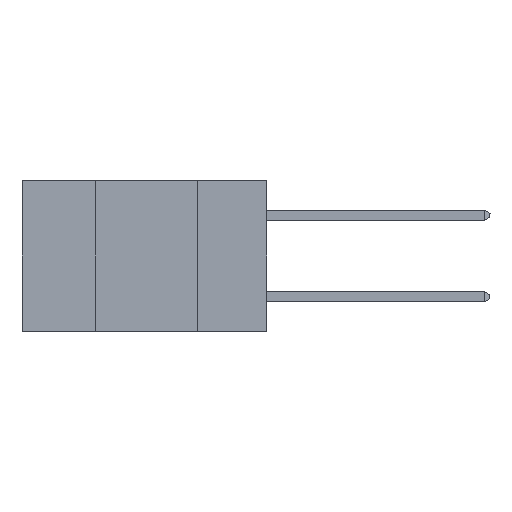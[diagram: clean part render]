
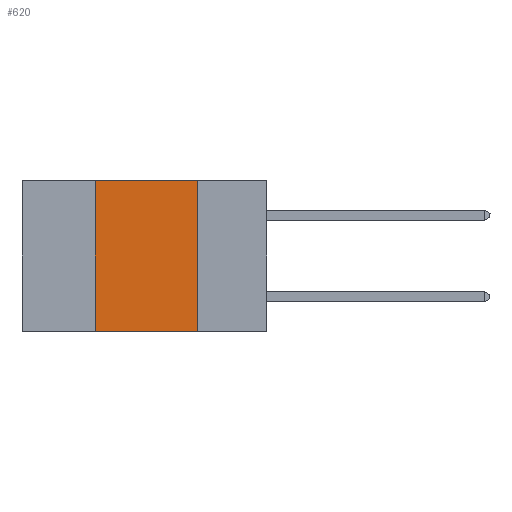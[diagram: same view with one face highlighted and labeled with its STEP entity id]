
A CAD part, left-side view. The second image highlights one B-rep face of the part: STEP entity #620.
In plain terms, the highlighted planar face has unit normal (-1, 0, 0).
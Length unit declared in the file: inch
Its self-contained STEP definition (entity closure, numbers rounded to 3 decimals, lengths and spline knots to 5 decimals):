
#140 = EDGE_CURVE ( 'NONE', #12637, #9687, #12186, .T. ) ;
#423 = EDGE_LOOP ( 'NONE', ( #9757, #9960, #8220, #6773 ) ) ;
#484 = CARTESIAN_POINT ( 'NONE',  ( 0., 0.42, -0.37 ) ) ;
#620 = ADVANCED_FACE ( 'NONE', ( #1312 ), #9565, .F. ) ;
#869 = EDGE_CURVE ( 'NONE', #1487, #12637, #4148, .T. ) ;
#1088 = CARTESIAN_POINT ( 'NONE',  ( 0., 0.17, 0. ) ) ;
#1160 = CARTESIAN_POINT ( 'NONE',  ( 0., 0.17, -0.37 ) ) ;
#1312 = FACE_OUTER_BOUND ( 'NONE', #423, .T. ) ;
#1487 = VERTEX_POINT ( 'NONE', #2853 ) ;
#2430 = LINE ( 'NONE', #8298, #12537 ) ;
#2853 = CARTESIAN_POINT ( 'NONE',  ( 0., 0.42, 0. ) ) ;
#3109 = CARTESIAN_POINT ( 'NONE',  ( 0., 0.6, -0.37 ) ) ;
#3334 = CARTESIAN_POINT ( 'NONE',  ( 0., 0.17, 0. ) ) ;
#3515 = DIRECTION ( 'NONE',  ( 1., 0., 0. ) ) ;
#4148 = LINE ( 'NONE', #11597, #9353 ) ;
#4589 = VERTEX_POINT ( 'NONE', #484 ) ;
#5140 = EDGE_CURVE ( 'NONE', #4589, #1487, #2430, .T. ) ;
#5810 = EDGE_CURVE ( 'NONE', #4589, #9687, #11799, .T. ) ;
#6275 = CARTESIAN_POINT ( 'NONE',  ( 0., 0.6, 0. ) ) ;
#6656 = DIRECTION ( 'NONE',  ( 0., 0., -1. ) ) ;
#6773 = ORIENTED_EDGE ( 'NONE', *, *, #5810, .T. ) ;
#7329 = DIRECTION ( 'NONE',  ( 0., 0., 1. ) ) ;
#8220 = ORIENTED_EDGE ( 'NONE', *, *, #5140, .F. ) ;
#8298 = CARTESIAN_POINT ( 'NONE',  ( 0., 0.42, 0. ) ) ;
#8971 = VECTOR ( 'NONE', #10925, 39.37008 ) ;
#9353 = VECTOR ( 'NONE', #10609, 39.37008 ) ;
#9565 = PLANE ( 'NONE',  #12101 ) ;
#9685 = VECTOR ( 'NONE', #10604, 39.37008 ) ;
#9687 = VERTEX_POINT ( 'NONE', #1160 ) ;
#9757 = ORIENTED_EDGE ( 'NONE', *, *, #140, .F. ) ;
#9960 = ORIENTED_EDGE ( 'NONE', *, *, #869, .F. ) ;
#10604 = DIRECTION ( 'NONE',  ( 0., 0., -1. ) ) ;
#10609 = DIRECTION ( 'NONE',  ( 0., -1., 0. ) ) ;
#10925 = DIRECTION ( 'NONE',  ( 0., -1., 0. ) ) ;
#11597 = CARTESIAN_POINT ( 'NONE',  ( 0., 0.6, 0. ) ) ;
#11799 = LINE ( 'NONE', #3109, #8971 ) ;
#12101 = AXIS2_PLACEMENT_3D ( 'NONE', #6275, #3515, #6656 ) ;
#12186 = LINE ( 'NONE', #1088, #9685 ) ;
#12537 = VECTOR ( 'NONE', #7329, 39.37008 ) ;
#12637 = VERTEX_POINT ( 'NONE', #3334 ) ;
